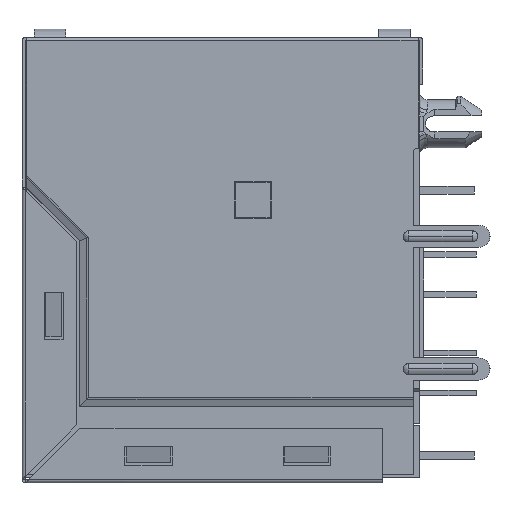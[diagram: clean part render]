
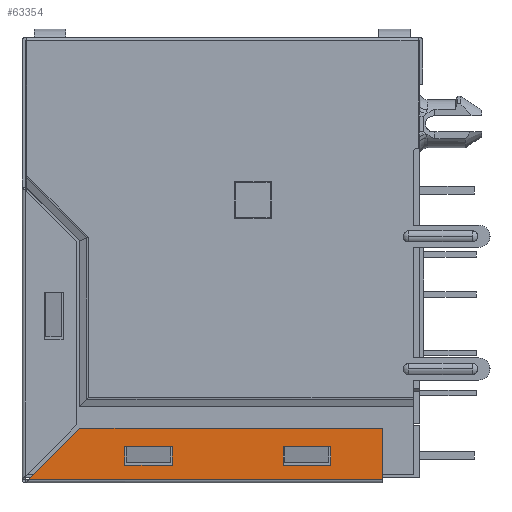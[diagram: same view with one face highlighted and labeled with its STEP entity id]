
A CAD part, left-side view. The second image highlights one B-rep face of the part: STEP entity #63354.
In plain terms, the highlighted planar face has unit normal (-1, 0, 0).
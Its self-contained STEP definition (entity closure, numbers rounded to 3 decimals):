
#114 = EDGE_CURVE ( 'NONE', #2301, #41915, #2413, .T. ) ;
#548 = FACE_BOUND ( 'NONE', #7595, .T. ) ;
#1349 = CARTESIAN_POINT ( 'NONE',  ( -31.88, 3.165, -25.58 ) ) ;
#1958 = CARTESIAN_POINT ( 'NONE',  ( -31.88, 6.165, -25.58 ) ) ;
#2301 = VERTEX_POINT ( 'NONE', #42690 ) ;
#2413 = B_SPLINE_CURVE_WITH_KNOTS ( 'NONE', 1,
 ( #6452, #42245 ),
 .UNSPECIFIED., .F., .F.,
 ( 2, 2 ),
 ( 0., 1. ),
 .UNSPECIFIED. ) ;
#3357 = DIRECTION ( 'NONE',  ( 0., -1., 0. ) ) ;
#3945 = EDGE_CURVE ( 'NONE', #52395, #61697, #70020, .T. ) ;
#4682 = EDGE_CURVE ( 'NONE', #66906, #43414, #31805, .T. ) ;
#5857 = CARTESIAN_POINT ( 'NONE',  ( -31.88, 6.165, -26.78 ) ) ;
#6452 = CARTESIAN_POINT ( 'NONE',  ( -31.88, -6.835, -25.58 ) ) ;
#7595 = EDGE_LOOP ( 'NONE', ( #42936, #38217, #78836, #56081 ) ) ;
#8798 = CARTESIAN_POINT ( 'NONE',  ( -31.88, -6.835, -26.78 ) ) ;
#8895 = CARTESIAN_POINT ( 'NONE',  ( -31.88, 12.245, -27.67 ) ) ;
#8910 = CARTESIAN_POINT ( 'NONE',  ( -31.88, 3.165, -25.58 ) ) ;
#13725 = CARTESIAN_POINT ( 'NONE',  ( -31.88, 6.165, -26.78 ) ) ;
#16293 = CARTESIAN_POINT ( 'NONE',  ( -31.88, -10.135, -24.43 ) ) ;
#16852 = ORIENTED_EDGE ( 'NONE', *, *, #60349, .T. ) ;
#16906 = EDGE_CURVE ( 'NONE', #48293, #67012, #34716, .T. ) ;
#17560 = CARTESIAN_POINT ( 'NONE',  ( -31.88, -3.835, -25.58 ) ) ;
#18319 = AXIS2_PLACEMENT_3D ( 'NONE', #53707, #71571, #40828 ) ;
#19274 = CARTESIAN_POINT ( 'NONE',  ( -31.88, -3.835, -25.58 ) ) ;
#19775 = CARTESIAN_POINT ( 'NONE',  ( -31.88, 3.165, -26.78 ) ) ;
#20925 = CARTESIAN_POINT ( 'NONE',  ( -31.88, 9.005, -24.43 ) ) ;
#21471 = ORIENTED_EDGE ( 'NONE', *, *, #56927, .T. ) ;
#23082 = ORIENTED_EDGE ( 'NONE', *, *, #49052, .T. ) ;
#23890 = VERTEX_POINT ( 'NONE', #53523 ) ;
#26473 = VERTEX_POINT ( 'NONE', #35103 ) ;
#27577 = VERTEX_POINT ( 'NONE', #37323 ) ;
#29314 = CARTESIAN_POINT ( 'NONE',  ( -31.88, -10.135, -27.67 ) ) ;
#30706 = B_SPLINE_CURVE_WITH_KNOTS ( 'NONE', 1,
 ( #16293, #52444 ),
 .UNSPECIFIED., .F., .F.,
 ( 2, 2 ),
 ( 0., 1. ),
 .UNSPECIFIED. ) ;
#31327 = CARTESIAN_POINT ( 'NONE',  ( -31.88, -10.135, -24.43 ) ) ;
#31805 = B_SPLINE_CURVE_WITH_KNOTS ( 'NONE', 1,
 ( #36023, #17560 ),
 .UNSPECIFIED., .F., .F.,
 ( 2, 2 ),
 ( 0., 1. ),
 .UNSPECIFIED. ) ;
#32142 = B_SPLINE_CURVE_WITH_KNOTS ( 'NONE', 1,
 ( #31327, #55203 ),
 .UNSPECIFIED., .F., .F.,
 ( 2, 2 ),
 ( 0., 1. ),
 .UNSPECIFIED. ) ;
#32517 = EDGE_CURVE ( 'NONE', #26473, #51657, #30706, .T. ) ;
#34716 = B_SPLINE_CURVE_WITH_KNOTS ( 'NONE', 1,
 ( #59782, #66193 ),
 .UNSPECIFIED., .F., .F.,
 ( 2, 2 ),
 ( 0., 1. ),
 .UNSPECIFIED. ) ;
#34962 = ORIENTED_EDGE ( 'NONE', *, *, #3945, .T. ) ;
#34975 = FACE_BOUND ( 'NONE', #72094, .T. ) ;
#35103 = CARTESIAN_POINT ( 'NONE',  ( -31.88, -10.135, -24.43 ) ) ;
#36023 = CARTESIAN_POINT ( 'NONE',  ( -31.88, -3.835, -26.78 ) ) ;
#37260 = VECTOR ( 'NONE', #3357, 1000. ) ;
#37323 = CARTESIAN_POINT ( 'NONE',  ( -31.88, 6.165, -26.78 ) ) ;
#38217 = ORIENTED_EDGE ( 'NONE', *, *, #50805, .T. ) ;
#39607 = FACE_OUTER_BOUND ( 'NONE', #45651, .T. ) ;
#39938 = CARTESIAN_POINT ( 'NONE',  ( -31.88, 1.055, -27.67 ) ) ;
#40828 = DIRECTION ( 'NONE',  ( 0., -1., 0. ) ) ;
#41915 = VERTEX_POINT ( 'NONE', #8798 ) ;
#42245 = CARTESIAN_POINT ( 'NONE',  ( -31.88, -6.835, -26.78 ) ) ;
#42690 = CARTESIAN_POINT ( 'NONE',  ( -31.88, -6.835, -25.58 ) ) ;
#42936 = ORIENTED_EDGE ( 'NONE', *, *, #114, .T. ) ;
#43414 = VERTEX_POINT ( 'NONE', #19274 ) ;
#44321 = EDGE_CURVE ( 'NONE', #43414, #2301, #69040, .T. ) ;
#45651 = EDGE_LOOP ( 'NONE', ( #59700, #56470, #34962, #16852 ) ) ;
#45901 = B_SPLINE_CURVE_WITH_KNOTS ( 'NONE', 1,
 ( #1349, #19775 ),
 .UNSPECIFIED., .F., .F.,
 ( 2, 2 ),
 ( 0., 1. ),
 .UNSPECIFIED. ) ;
#46343 = B_SPLINE_CURVE_WITH_KNOTS ( 'NONE', 1,
 ( #13725, #1958 ),
 .UNSPECIFIED., .F., .F.,
 ( 2, 2 ),
 ( 0., 1. ),
 .UNSPECIFIED. ) ;
#48293 = VERTEX_POINT ( 'NONE', #54174 ) ;
#49052 = EDGE_CURVE ( 'NONE', #67012, #23890, #45901, .T. ) ;
#49584 = ORIENTED_EDGE ( 'NONE', *, *, #58865, .T. ) ;
#50805 = EDGE_CURVE ( 'NONE', #41915, #66906, #72893, .T. ) ;
#50947 = CARTESIAN_POINT ( 'NONE',  ( -31.88, -3.835, -26.78 ) ) ;
#51657 = VERTEX_POINT ( 'NONE', #29314 ) ;
#52395 = VERTEX_POINT ( 'NONE', #60830 ) ;
#52444 = CARTESIAN_POINT ( 'NONE',  ( -31.88, -10.135, -27.67 ) ) ;
#53181 = PLANE ( 'NONE',  #18319 ) ;
#53523 = CARTESIAN_POINT ( 'NONE',  ( -31.88, 3.165, -26.78 ) ) ;
#53707 = CARTESIAN_POINT ( 'NONE',  ( -31.88, 12.693, -27.79 ) ) ;
#54174 = CARTESIAN_POINT ( 'NONE',  ( -31.88, 6.165, -25.58 ) ) ;
#54977 = CARTESIAN_POINT ( 'NONE',  ( -31.88, -3.835, -26.78 ) ) ;
#55203 = CARTESIAN_POINT ( 'NONE',  ( -31.88, 9.005, -24.43 ) ) ;
#56081 = ORIENTED_EDGE ( 'NONE', *, *, #44321, .T. ) ;
#56448 = ORIENTED_EDGE ( 'NONE', *, *, #16906, .T. ) ;
#56470 = ORIENTED_EDGE ( 'NONE', *, *, #60616, .T. ) ;
#56927 = EDGE_CURVE ( 'NONE', #23890, #27577, #66488, .T. ) ;
#58865 = EDGE_CURVE ( 'NONE', #27577, #48293, #46343, .T. ) ;
#59700 = ORIENTED_EDGE ( 'NONE', *, *, #32517, .F. ) ;
#59782 = CARTESIAN_POINT ( 'NONE',  ( -31.88, 6.165, -25.58 ) ) ;
#60349 = EDGE_CURVE ( 'NONE', #61697, #51657, #68882, .T. ) ;
#60616 = EDGE_CURVE ( 'NONE', #26473, #52395, #32142, .T. ) ;
#60642 = CARTESIAN_POINT ( 'NONE',  ( -31.88, 12.245, -27.67 ) ) ;
#60830 = CARTESIAN_POINT ( 'NONE',  ( -31.88, 9.005, -24.43 ) ) ;
#61435 = CARTESIAN_POINT ( 'NONE',  ( -31.88, 3.165, -26.78 ) ) ;
#61697 = VERTEX_POINT ( 'NONE', #60642 ) ;
#63354 = ADVANCED_FACE ( 'NONE', ( #39607, #548, #34975 ), #53181, .T. ) ;
#66193 = CARTESIAN_POINT ( 'NONE',  ( -31.88, 3.165, -25.58 ) ) ;
#66348 = CARTESIAN_POINT ( 'NONE',  ( -31.88, -3.835, -25.58 ) ) ;
#66488 = B_SPLINE_CURVE_WITH_KNOTS ( 'NONE', 1,
 ( #61435, #5857 ),
 .UNSPECIFIED., .F., .F.,
 ( 2, 2 ),
 ( 0., 1. ),
 .UNSPECIFIED. ) ;
#66906 = VERTEX_POINT ( 'NONE', #50947 ) ;
#67012 = VERTEX_POINT ( 'NONE', #8910 ) ;
#67500 = CARTESIAN_POINT ( 'NONE',  ( -31.88, -6.835, -26.78 ) ) ;
#68882 = LINE ( 'NONE', #39938, #37260 ) ;
#69040 = B_SPLINE_CURVE_WITH_KNOTS ( 'NONE', 1,
 ( #66348, #78285 ),
 .UNSPECIFIED., .F., .F.,
 ( 2, 2 ),
 ( 0., 1. ),
 .UNSPECIFIED. ) ;
#70020 = B_SPLINE_CURVE_WITH_KNOTS ( 'NONE', 1,
 ( #20925, #8895 ),
 .UNSPECIFIED., .F., .F.,
 ( 2, 2 ),
 ( 0., 1. ),
 .UNSPECIFIED. ) ;
#71571 = DIRECTION ( 'NONE',  ( -1., 0., 0. ) ) ;
#72094 = EDGE_LOOP ( 'NONE', ( #23082, #21471, #49584, #56448 ) ) ;
#72893 = B_SPLINE_CURVE_WITH_KNOTS ( 'NONE', 1,
 ( #67500, #54977 ),
 .UNSPECIFIED., .F., .F.,
 ( 2, 2 ),
 ( 0., 1. ),
 .UNSPECIFIED. ) ;
#78285 = CARTESIAN_POINT ( 'NONE',  ( -31.88, -6.835, -25.58 ) ) ;
#78836 = ORIENTED_EDGE ( 'NONE', *, *, #4682, .T. ) ;
